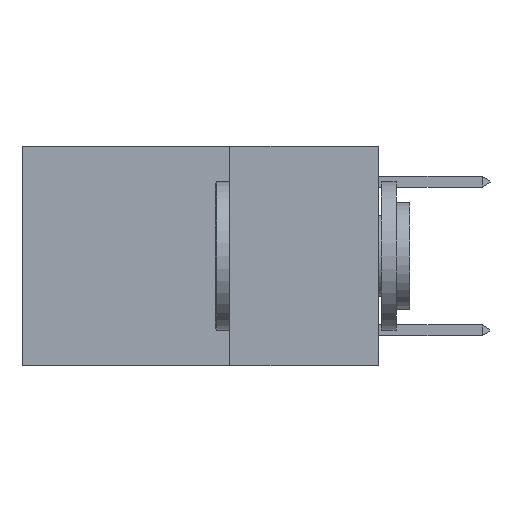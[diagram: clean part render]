
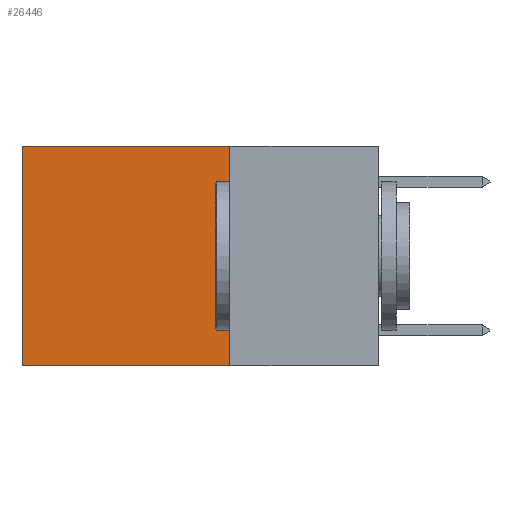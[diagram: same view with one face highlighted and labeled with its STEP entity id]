
A CAD part, left-side view. The second image highlights one B-rep face of the part: STEP entity #26446.
In plain terms, the highlighted planar face has unit normal (-1, 0, 0).
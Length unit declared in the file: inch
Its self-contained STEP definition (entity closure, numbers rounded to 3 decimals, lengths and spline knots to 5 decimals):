
#1047 = VERTEX_POINT ( 'NONE', #19259 ) ;
#2076 = LINE ( 'NONE', #6481, #14050 ) ;
#2815 = EDGE_CURVE ( 'NONE', #27762, #18262, #25491, .T. ) ;
#2939 = EDGE_LOOP ( 'NONE', ( #17151, #22069, #20204, #25510 ) ) ;
#4301 = LINE ( 'NONE', #11152, #27261 ) ;
#6481 = CARTESIAN_POINT ( 'NONE',  ( 0.2625, 0.25, 0. ) ) ;
#7499 = EDGE_CURVE ( 'NONE', #18262, #7840, #4301, .T. ) ;
#7840 = VERTEX_POINT ( 'NONE', #16817 ) ;
#8248 = CARTESIAN_POINT ( 'NONE',  ( 0.2625, 0.25, -0.37 ) ) ;
#8278 = EDGE_CURVE ( 'NONE', #27762, #1047, #2076, .T. ) ;
#9793 = PLANE ( 'NONE',  #25323 ) ;
#10365 = CARTESIAN_POINT ( 'NONE',  ( 0.2625, 0.25, 0. ) ) ;
#11152 = CARTESIAN_POINT ( 'NONE',  ( 0.2625, 0.25, -0.37 ) ) ;
#11648 = DIRECTION ( 'NONE',  ( 0., 0., -1. ) ) ;
#13781 = DIRECTION ( 'NONE',  ( 1., 0., 0. ) ) ;
#14050 = VECTOR ( 'NONE', #18883, 39.37008 ) ;
#14190 = CARTESIAN_POINT ( 'NONE',  ( 0.2625, 0.25, 0. ) ) ;
#14952 = LINE ( 'NONE', #16656, #16692 ) ;
#16656 = CARTESIAN_POINT ( 'NONE',  ( 0.2625, 0.6, 0. ) ) ;
#16692 = VECTOR ( 'NONE', #23333, 39.37008 ) ;
#16817 = CARTESIAN_POINT ( 'NONE',  ( 0.2625, 0.6, -0.37 ) ) ;
#17151 = ORIENTED_EDGE ( 'NONE', *, *, #26084, .T. ) ;
#17419 = DIRECTION ( 'NONE',  ( 0., 1., 0. ) ) ;
#18262 = VERTEX_POINT ( 'NONE', #8248 ) ;
#18883 = DIRECTION ( 'NONE',  ( 0., 1., 0. ) ) ;
#19259 = CARTESIAN_POINT ( 'NONE',  ( 0.2625, 0.6, 0. ) ) ;
#20204 = ORIENTED_EDGE ( 'NONE', *, *, #2815, .F. ) ;
#20482 = FACE_OUTER_BOUND ( 'NONE', #2939, .T. ) ;
#22069 = ORIENTED_EDGE ( 'NONE', *, *, #7499, .F. ) ;
#22901 = VECTOR ( 'NONE', #23346, 39.37008 ) ;
#23073 = CARTESIAN_POINT ( 'NONE',  ( 0.2625, 0.25, 0. ) ) ;
#23333 = DIRECTION ( 'NONE',  ( 0., 0., -1. ) ) ;
#23346 = DIRECTION ( 'NONE',  ( 0., 0., -1. ) ) ;
#25323 = AXIS2_PLACEMENT_3D ( 'NONE', #14190, #13781, #11648 ) ;
#25491 = LINE ( 'NONE', #23073, #22901 ) ;
#25510 = ORIENTED_EDGE ( 'NONE', *, *, #8278, .T. ) ;
#26084 = EDGE_CURVE ( 'NONE', #1047, #7840, #14952, .T. ) ;
#26446 = ADVANCED_FACE ( 'NONE', ( #20482 ), #9793, .F. ) ;
#27261 = VECTOR ( 'NONE', #17419, 39.37008 ) ;
#27762 = VERTEX_POINT ( 'NONE', #10365 ) ;
